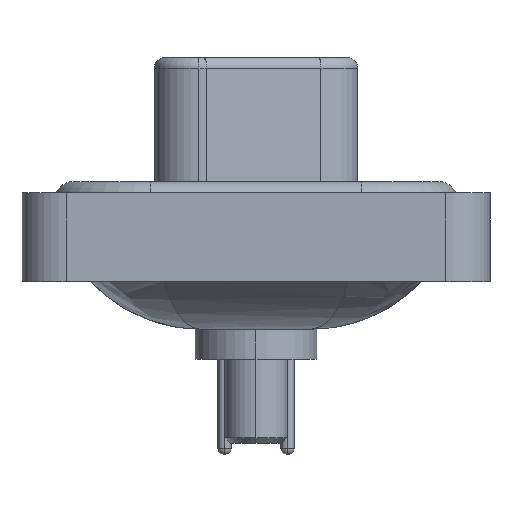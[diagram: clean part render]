
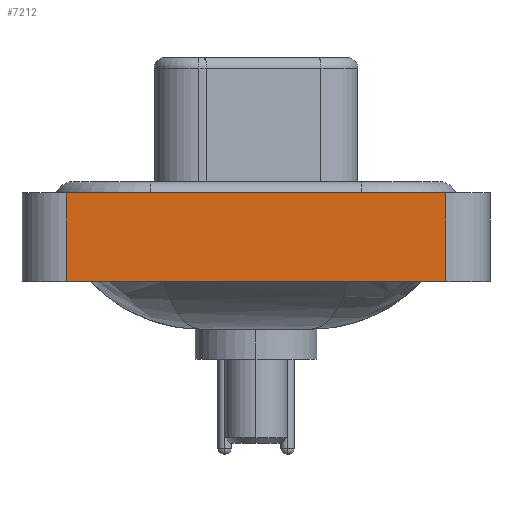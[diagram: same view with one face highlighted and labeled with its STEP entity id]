
A CAD part, left-side view. The second image highlights one B-rep face of the part: STEP entity #7212.
In plain terms, the highlighted planar face has unit normal (-1, 0, 0).
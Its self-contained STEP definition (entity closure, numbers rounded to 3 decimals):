
#354 = EDGE_CURVE ( 'NONE', #3137, #912, #11092, .T. ) ;
#802 = CARTESIAN_POINT ( 'NONE',  ( -7.35, -8.55, -3.6 ) ) ;
#912 = VERTEX_POINT ( 'NONE', #20701 ) ;
#1290 = EDGE_CURVE ( 'NONE', #10204, #912, #21940, .T. ) ;
#2145 = CARTESIAN_POINT ( 'NONE',  ( -7.35, -8.55, -3.6 ) ) ;
#2589 = DIRECTION ( 'NONE',  ( 0., -1., 0. ) ) ;
#2712 = LINE ( 'NONE', #4708, #11027 ) ;
#3137 = VERTEX_POINT ( 'NONE', #5889 ) ;
#3596 = LINE ( 'NONE', #12468, #16413 ) ;
#4139 = ORIENTED_EDGE ( 'NONE', *, *, #1290, .T. ) ;
#4372 = EDGE_CURVE ( 'NONE', #21920, #10204, #2712, .T. ) ;
#4708 = CARTESIAN_POINT ( 'NONE',  ( -7.35, -8.55, -3.6 ) ) ;
#5879 = FACE_OUTER_BOUND ( 'NONE', #11300, .T. ) ;
#5889 = CARTESIAN_POINT ( 'NONE',  ( -7.35, 8.55, 0.4 ) ) ;
#6040 = DIRECTION ( 'NONE',  ( 0., 0., 1. ) ) ;
#7212 = ADVANCED_FACE ( 'NONE', ( #5879 ), #11003, .T. ) ;
#9813 = DIRECTION ( 'NONE',  ( 0., -1., 0. ) ) ;
#10204 = VERTEX_POINT ( 'NONE', #802 ) ;
#10996 = ORIENTED_EDGE ( 'NONE', *, *, #22475, .F. ) ;
#11003 = PLANE ( 'NONE',  #21911 ) ;
#11027 = VECTOR ( 'NONE', #9813, 1000. ) ;
#11037 = CARTESIAN_POINT ( 'NONE',  ( -7.35, -8.55, -3.6 ) ) ;
#11092 = LINE ( 'NONE', #14707, #14965 ) ;
#11300 = EDGE_LOOP ( 'NONE', ( #4139, #15273, #10996, #16486 ) ) ;
#12467 = VECTOR ( 'NONE', #6040, 1000. ) ;
#12468 = CARTESIAN_POINT ( 'NONE',  ( -7.35, 8.55, -3.6 ) ) ;
#13001 = DIRECTION ( 'NONE',  ( -1., 0., 0. ) ) ;
#14707 = CARTESIAN_POINT ( 'NONE',  ( -7.35, -8.55, 0.4 ) ) ;
#14965 = VECTOR ( 'NONE', #2589, 1000. ) ;
#15273 = ORIENTED_EDGE ( 'NONE', *, *, #354, .F. ) ;
#16413 = VECTOR ( 'NONE', #17545, 1000. ) ;
#16486 = ORIENTED_EDGE ( 'NONE', *, *, #4372, .T. ) ;
#17545 = DIRECTION ( 'NONE',  ( 0., 0., 1. ) ) ;
#18855 = CARTESIAN_POINT ( 'NONE',  ( -7.35, 8.55, -3.6 ) ) ;
#20062 = DIRECTION ( 'NONE',  ( 0., 0., 1. ) ) ;
#20701 = CARTESIAN_POINT ( 'NONE',  ( -7.35, -8.55, 0.4 ) ) ;
#21911 = AXIS2_PLACEMENT_3D ( 'NONE', #2145, #13001, #20062 ) ;
#21920 = VERTEX_POINT ( 'NONE', #18855 ) ;
#21940 = LINE ( 'NONE', #11037, #12467 ) ;
#22475 = EDGE_CURVE ( 'NONE', #21920, #3137, #3596, .T. ) ;
